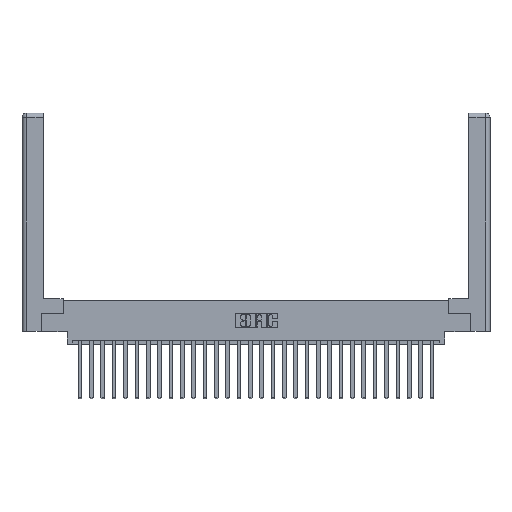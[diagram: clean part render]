
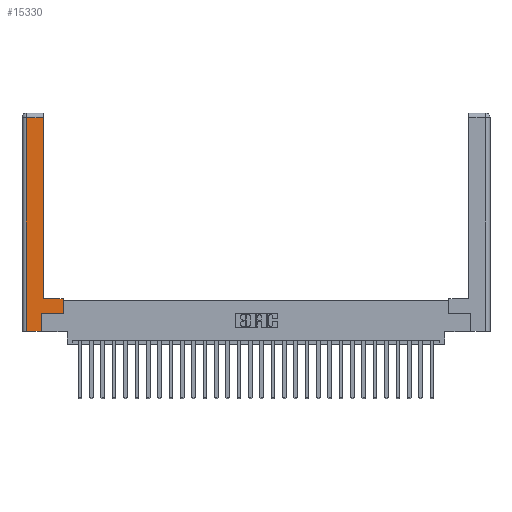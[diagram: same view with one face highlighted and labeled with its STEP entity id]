
A CAD part, top view. The second image highlights one B-rep face of the part: STEP entity #15330.
In plain terms, the highlighted planar face has unit normal (0, 0, 1).
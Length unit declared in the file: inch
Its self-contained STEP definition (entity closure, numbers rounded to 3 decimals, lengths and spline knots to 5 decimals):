
#68 = DIRECTION ( 'NONE',  ( -1., 0., 0. ) ) ;
#275 = ORIENTED_EDGE ( 'NONE', *, *, #8645, .T. ) ;
#2132 = EDGE_LOOP ( 'NONE', ( #8752, #3672, #19219, #275, #23497, #28317, #22315, #15003 ) ) ;
#3672 = ORIENTED_EDGE ( 'NONE', *, *, #12338, .T. ) ;
#3708 = DIRECTION ( 'NONE',  ( 0., 0., -1. ) ) ;
#3802 = EDGE_CURVE ( 'NONE', #4964, #11355, #13163, .T. ) ;
#3818 = VERTEX_POINT ( 'NONE', #27267 ) ;
#3942 = DIRECTION ( 'NONE',  ( 0., 1., 0. ) ) ;
#4154 = CARTESIAN_POINT ( 'NONE',  ( 0.0615, 0., 0. ) ) ;
#4716 = CARTESIAN_POINT ( 'NONE',  ( 0.565, 0.245, 0. ) ) ;
#4964 = VERTEX_POINT ( 'NONE', #7980 ) ;
#6332 = VECTOR ( 'NONE', #25395, 39.37008 ) ;
#6607 = EDGE_CURVE ( 'NONE', #11355, #14372, #16711, .T. ) ;
#6637 = CARTESIAN_POINT ( 'NONE',  ( 0.295, 0.45, 0. ) ) ;
#6944 = VECTOR ( 'NONE', #3942, 39.37008 ) ;
#7776 = CARTESIAN_POINT ( 'NONE',  ( 0.0615, 2.94, 0. ) ) ;
#7980 = CARTESIAN_POINT ( 'NONE',  ( 0.565, 0.245, 0. ) ) ;
#8645 = EDGE_CURVE ( 'NONE', #27528, #14705, #23443, .T. ) ;
#8752 = ORIENTED_EDGE ( 'NONE', *, *, #23954, .T. ) ;
#9177 = CARTESIAN_POINT ( 'NONE',  ( 0.0615, 0., 0. ) ) ;
#9196 = DIRECTION ( 'NONE',  ( 0., 1., 0. ) ) ;
#11229 = CARTESIAN_POINT ( 'NONE',  ( 0.565, 0.45, 0. ) ) ;
#11314 = DIRECTION ( 'NONE',  ( 0., -1., 0. ) ) ;
#11355 = VERTEX_POINT ( 'NONE', #11229 ) ;
#11800 = VECTOR ( 'NONE', #18065, 39.37008 ) ;
#12338 = EDGE_CURVE ( 'NONE', #21325, #3818, #24008, .T. ) ;
#12866 = VECTOR ( 'NONE', #11314, 39.37008 ) ;
#13163 = LINE ( 'NONE', #20235, #20389 ) ;
#13802 = CARTESIAN_POINT ( 'NONE',  ( 0.265, 0.245, 0. ) ) ;
#14372 = VERTEX_POINT ( 'NONE', #17533 ) ;
#14705 = VERTEX_POINT ( 'NONE', #24753 ) ;
#15003 = ORIENTED_EDGE ( 'NONE', *, *, #6607, .T. ) ;
#15330 = ADVANCED_FACE ( 'NONE', ( #28017 ), #17054, .F. ) ;
#16711 = LINE ( 'NONE', #6637, #17755 ) ;
#17027 = EDGE_CURVE ( 'NONE', #3818, #27528, #21118, .T. ) ;
#17054 = PLANE ( 'NONE',  #22795 ) ;
#17533 = CARTESIAN_POINT ( 'NONE',  ( 0.295, 0.45, 0. ) ) ;
#17755 = VECTOR ( 'NONE', #68, 39.37008 ) ;
#18065 = DIRECTION ( 'NONE',  ( 0., 1., 0. ) ) ;
#18767 = LINE ( 'NONE', #23905, #6944 ) ;
#19219 = ORIENTED_EDGE ( 'NONE', *, *, #17027, .T. ) ;
#19910 = DIRECTION ( 'NONE',  ( 1., 0., 0. ) ) ;
#19988 = VERTEX_POINT ( 'NONE', #13802 ) ;
#20211 = CARTESIAN_POINT ( 'NONE',  ( 0.265, 0., 0. ) ) ;
#20235 = CARTESIAN_POINT ( 'NONE',  ( 0.565, 0.45, 0. ) ) ;
#20389 = VECTOR ( 'NONE', #9196, 39.37008 ) ;
#21118 = LINE ( 'NONE', #9177, #12866 ) ;
#21325 = VERTEX_POINT ( 'NONE', #28622 ) ;
#22315 = ORIENTED_EDGE ( 'NONE', *, *, #3802, .T. ) ;
#22795 = AXIS2_PLACEMENT_3D ( 'NONE', #27744, #3708, #25514 ) ;
#23242 = EDGE_CURVE ( 'NONE', #14705, #19988, #18767, .T. ) ;
#23443 = LINE ( 'NONE', #20211, #26906 ) ;
#23496 = VECTOR ( 'NONE', #24775, 39.37008 ) ;
#23497 = ORIENTED_EDGE ( 'NONE', *, *, #23242, .T. ) ;
#23905 = CARTESIAN_POINT ( 'NONE',  ( 0.265, 0.245, 0. ) ) ;
#23954 = EDGE_CURVE ( 'NONE', #14372, #21325, #24931, .T. ) ;
#24008 = LINE ( 'NONE', #7776, #6332 ) ;
#24276 = EDGE_CURVE ( 'NONE', #19988, #4964, #24563, .T. ) ;
#24563 = LINE ( 'NONE', #4716, #23496 ) ;
#24753 = CARTESIAN_POINT ( 'NONE',  ( 0.265, 0., 0. ) ) ;
#24775 = DIRECTION ( 'NONE',  ( 1., 0., 0. ) ) ;
#24931 = LINE ( 'NONE', #26807, #11800 ) ;
#25395 = DIRECTION ( 'NONE',  ( -1., 0., 0. ) ) ;
#25514 = DIRECTION ( 'NONE',  ( -1., 0., 0. ) ) ;
#26807 = CARTESIAN_POINT ( 'NONE',  ( 0.295, 3., 0. ) ) ;
#26906 = VECTOR ( 'NONE', #19910, 39.37008 ) ;
#27267 = CARTESIAN_POINT ( 'NONE',  ( 0.0615, 2.94, 0. ) ) ;
#27528 = VERTEX_POINT ( 'NONE', #4154 ) ;
#27744 = CARTESIAN_POINT ( 'NONE',  ( 0., 0., 0. ) ) ;
#28017 = FACE_OUTER_BOUND ( 'NONE', #2132, .T. ) ;
#28317 = ORIENTED_EDGE ( 'NONE', *, *, #24276, .T. ) ;
#28622 = CARTESIAN_POINT ( 'NONE',  ( 0.295, 2.94, 0. ) ) ;
